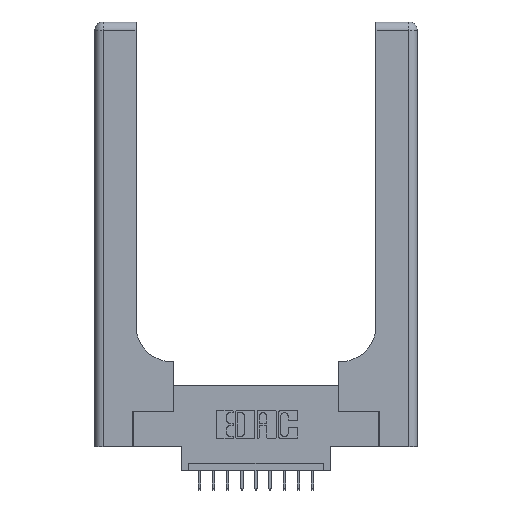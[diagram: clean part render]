
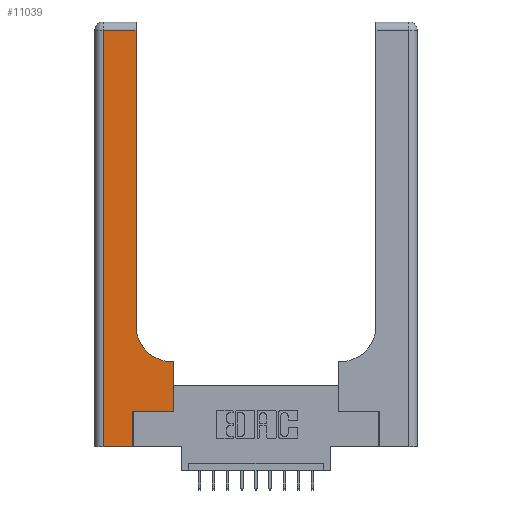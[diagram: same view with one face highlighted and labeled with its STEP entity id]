
A CAD part, top view. The second image highlights one B-rep face of the part: STEP entity #11039.
In plain terms, the highlighted planar face has unit normal (0, 0, 1).
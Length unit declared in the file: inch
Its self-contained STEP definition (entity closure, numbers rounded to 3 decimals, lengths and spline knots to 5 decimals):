
#306 = EDGE_CURVE ( 'NONE', #1807, #13319, #9385, .T. ) ;
#1512 = VECTOR ( 'NONE', #15015, 39.37008 ) ;
#1670 = CARTESIAN_POINT ( 'NONE',  ( 0.5585, 0.25, 0.37 ) ) ;
#1807 = VERTEX_POINT ( 'NONE', #3745 ) ;
#1968 = EDGE_CURVE ( 'NONE', #14769, #3848, #3916, .T. ) ;
#2001 = CARTESIAN_POINT ( 'NONE',  ( 0., 0., 0.37 ) ) ;
#2006 = CARTESIAN_POINT ( 'NONE',  ( 0.2915, 0.6, 0.37 ) ) ;
#2020 = ORIENTED_EDGE ( 'NONE', *, *, #16169, .T. ) ;
#2168 = LINE ( 'NONE', #2001, #4818 ) ;
#3033 = LINE ( 'NONE', #2006, #12131 ) ;
#3486 = FACE_OUTER_BOUND ( 'NONE', #13703, .T. ) ;
#3650 = CARTESIAN_POINT ( 'NONE',  ( 0., 3., 0.37 ) ) ;
#3745 = CARTESIAN_POINT ( 'NONE',  ( 0.5415, 0.6, 0.37 ) ) ;
#3848 = VERTEX_POINT ( 'NONE', #6562 ) ;
#3899 = CARTESIAN_POINT ( 'NONE',  ( 0.269, 0.25, 0.37 ) ) ;
#3916 = LINE ( 'NONE', #6512, #4502 ) ;
#3953 = ORIENTED_EDGE ( 'NONE', *, *, #1968, .T. ) ;
#4188 = VECTOR ( 'NONE', #9456, 39.37008 ) ;
#4284 = AXIS2_PLACEMENT_3D ( 'NONE', #13860, #13691, #6306 ) ;
#4336 = VERTEX_POINT ( 'NONE', #8976 ) ;
#4502 = VECTOR ( 'NONE', #10542, 39.37008 ) ;
#4768 = EDGE_CURVE ( 'NONE', #11012, #1807, #3033, .T. ) ;
#4818 = VECTOR ( 'NONE', #15216, 39.37008 ) ;
#4911 = ORIENTED_EDGE ( 'NONE', *, *, #13672, .T. ) ;
#5109 = CARTESIAN_POINT ( 'NONE',  ( 0.06, 3., 0.37 ) ) ;
#6006 = CARTESIAN_POINT ( 'NONE',  ( 0.5585, 0.6, 0.37 ) ) ;
#6208 = CARTESIAN_POINT ( 'NONE',  ( 0.2915, 3., 0.37 ) ) ;
#6306 = DIRECTION ( 'NONE',  ( 1., 0., 0. ) ) ;
#6512 = CARTESIAN_POINT ( 'NONE',  ( 0., 2.94, 0.37 ) ) ;
#6562 = CARTESIAN_POINT ( 'NONE',  ( 0.06, 2.94, 0.37 ) ) ;
#6740 = LINE ( 'NONE', #7679, #11145 ) ;
#6872 = VECTOR ( 'NONE', #8897, 39.37008 ) ;
#6978 = DIRECTION ( 'NONE',  ( -1., 0., 0. ) ) ;
#7198 = CARTESIAN_POINT ( 'NONE',  ( 0.2915, 2.94, 0.37 ) ) ;
#7426 = DIRECTION ( 'NONE',  ( -1., 0., 0. ) ) ;
#7623 = LINE ( 'NONE', #5109, #1512 ) ;
#7679 = CARTESIAN_POINT ( 'NONE',  ( 0.269, 0.25, 0.37 ) ) ;
#7761 = EDGE_CURVE ( 'NONE', #4336, #15827, #14209, .T. ) ;
#7899 = CARTESIAN_POINT ( 'NONE',  ( 0.269, 0., 0.37 ) ) ;
#8897 = DIRECTION ( 'NONE',  ( 0., 1., 0. ) ) ;
#8976 = CARTESIAN_POINT ( 'NONE',  ( 0.269, 0., 0.37 ) ) ;
#9025 = AXIS2_PLACEMENT_3D ( 'NONE', #3650, #10038, #7426 ) ;
#9051 = ORIENTED_EDGE ( 'NONE', *, *, #9724, .T. ) ;
#9385 = CIRCLE ( 'NONE', #4284, 0.25 ) ;
#9456 = DIRECTION ( 'NONE',  ( 0., 1., 0. ) ) ;
#9684 = ORIENTED_EDGE ( 'NONE', *, *, #7761, .T. ) ;
#9724 = EDGE_CURVE ( 'NONE', #15827, #12737, #6740, .T. ) ;
#10038 = DIRECTION ( 'NONE',  ( 0., 0., -1. ) ) ;
#10542 = DIRECTION ( 'NONE',  ( -1., 0., 0. ) ) ;
#11012 = VERTEX_POINT ( 'NONE', #6006 ) ;
#11039 = ADVANCED_FACE ( 'NONE', ( #3486 ), #12736, .F. ) ;
#11145 = VECTOR ( 'NONE', #14070, 39.37008 ) ;
#11361 = ORIENTED_EDGE ( 'NONE', *, *, #4768, .T. ) ;
#12064 = CARTESIAN_POINT ( 'NONE',  ( 0.5585, 0.25, 0.37 ) ) ;
#12131 = VECTOR ( 'NONE', #6978, 39.37008 ) ;
#12301 = ORIENTED_EDGE ( 'NONE', *, *, #13270, .T. ) ;
#12430 = VECTOR ( 'NONE', #15478, 39.37008 ) ;
#12553 = EDGE_CURVE ( 'NONE', #12737, #11012, #15767, .T. ) ;
#12736 = PLANE ( 'NONE',  #9025 ) ;
#12737 = VERTEX_POINT ( 'NONE', #1670 ) ;
#12770 = LINE ( 'NONE', #6208, #6872 ) ;
#13171 = CARTESIAN_POINT ( 'NONE',  ( 0.2915, 0.85, 0.37 ) ) ;
#13270 = EDGE_CURVE ( 'NONE', #13319, #14769, #12770, .T. ) ;
#13319 = VERTEX_POINT ( 'NONE', #13171 ) ;
#13571 = ORIENTED_EDGE ( 'NONE', *, *, #306, .T. ) ;
#13672 = EDGE_CURVE ( 'NONE', #3848, #16631, #7623, .T. ) ;
#13691 = DIRECTION ( 'NONE',  ( 0., 0., -1. ) ) ;
#13703 = EDGE_LOOP ( 'NONE', ( #12301, #3953, #4911, #2020, #9684, #9051, #13910, #11361, #13571 ) ) ;
#13860 = CARTESIAN_POINT ( 'NONE',  ( 0.5415, 0.85, 0.37 ) ) ;
#13910 = ORIENTED_EDGE ( 'NONE', *, *, #12553, .T. ) ;
#14070 = DIRECTION ( 'NONE',  ( 1., 0., 0. ) ) ;
#14209 = LINE ( 'NONE', #7899, #12430 ) ;
#14769 = VERTEX_POINT ( 'NONE', #7198 ) ;
#15015 = DIRECTION ( 'NONE',  ( 0., -1., 0. ) ) ;
#15216 = DIRECTION ( 'NONE',  ( 1., 0., 0. ) ) ;
#15478 = DIRECTION ( 'NONE',  ( 0., 1., 0. ) ) ;
#15754 = CARTESIAN_POINT ( 'NONE',  ( 0.06, 0., 0.37 ) ) ;
#15767 = LINE ( 'NONE', #12064, #4188 ) ;
#15827 = VERTEX_POINT ( 'NONE', #3899 ) ;
#16169 = EDGE_CURVE ( 'NONE', #16631, #4336, #2168, .T. ) ;
#16631 = VERTEX_POINT ( 'NONE', #15754 ) ;
